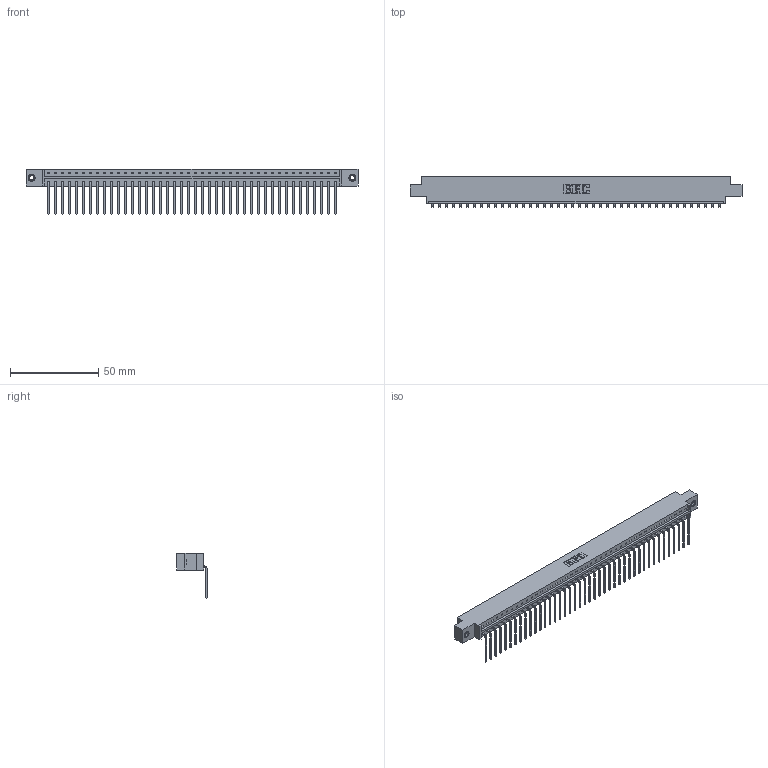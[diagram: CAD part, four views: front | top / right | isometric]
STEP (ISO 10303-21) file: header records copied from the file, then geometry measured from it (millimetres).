
FILE_DESCRIPTION (( 'STEP AP203' ), '1' );
FILE_NAME ('333-042-559-607.STEP', '2018-08-03T19:46:45', ( '' ), ( '' ), 'SwSTEP 2.0', 'SolidWorks 2016', '' );
FILE_SCHEMA (( 'CONFIG_CONTROL_DESIGN' ));
Length unit declared in the file: inch
Products named in the file (4): 345-292-001_558 559 Tail - 1; 345-250-001_345-250-005-103; 333-042-559-607; 333 Part_Offset - .156 Dia - TI
Assembly tree (45 placements, depth 2):
  333-042-559-607
    333 Part_Offset - .156 Dia - TI
    345-292-001_558 559 Tail - 1  x42
    345-250-001_345-250-005-103  x2
Bounding box: 187.96 x 17.09 x 25.53 mm (x, y, z)
Volume: 18812.7 mm3; surface area: 21448.7 mm2
Topology: 45 solids, 45 shells, 2698 faces, 8103 edges, 5338 vertices
Faces by surface type: plane 1954, cylinder 728, cone 12, torus 4
Entity records: 27078 total; most frequent: CARTESIAN_POINT 4655, ORIENTED_EDGE 4626, DIRECTION 3959, EDGE_CURVE 2313, LINE 2165, VECTOR 2165, VERTEX_POINT 1536, AXIS2_PLACEMENT_3D 897
